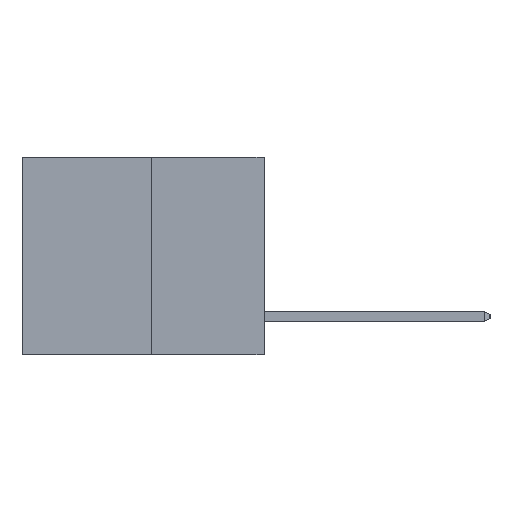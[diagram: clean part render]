
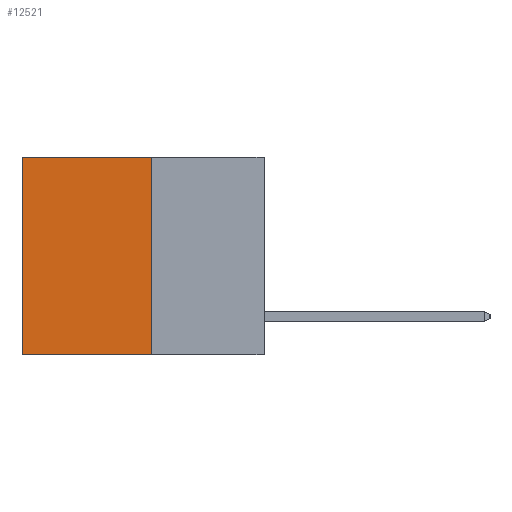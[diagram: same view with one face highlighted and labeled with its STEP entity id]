
A CAD part, left-side view. The second image highlights one B-rep face of the part: STEP entity #12521.
In plain terms, the highlighted planar face has unit normal (-1, 0, 0).
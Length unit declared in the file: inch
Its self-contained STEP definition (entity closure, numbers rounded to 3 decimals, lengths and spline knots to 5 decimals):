
#630 = DIRECTION ( 'NONE',  ( 1., 0., 0. ) ) ;
#1198 = CARTESIAN_POINT ( 'NONE',  ( 0.3165, 0.6, 0. ) ) ;
#1320 = EDGE_CURVE ( 'NONE', #2112, #13241, #15184, .T. ) ;
#1486 = CARTESIAN_POINT ( 'NONE',  ( 0.3165, 0.6, -0.49 ) ) ;
#2061 = DIRECTION ( 'NONE',  ( 0., 0., -1. ) ) ;
#2112 = VERTEX_POINT ( 'NONE', #1198 ) ;
#2833 = DIRECTION ( 'NONE',  ( 0., 1., 0. ) ) ;
#2996 = DIRECTION ( 'NONE',  ( 0., 0., -1. ) ) ;
#3142 = VERTEX_POINT ( 'NONE', #16560 ) ;
#4408 = EDGE_CURVE ( 'NONE', #3142, #2112, #5765, .T. ) ;
#5420 = CARTESIAN_POINT ( 'NONE',  ( 0.3165, 0.6, -0.49 ) ) ;
#5765 = LINE ( 'NONE', #13756, #8947 ) ;
#5780 = ORIENTED_EDGE ( 'NONE', *, *, #1320, .T. ) ;
#6660 = EDGE_CURVE ( 'NONE', #3142, #11105, #7778, .T. ) ;
#6782 = ORIENTED_EDGE ( 'NONE', *, *, #6660, .F. ) ;
#7140 = VECTOR ( 'NONE', #2061, 39.37008 ) ;
#7445 = AXIS2_PLACEMENT_3D ( 'NONE', #12868, #630, #7494 ) ;
#7494 = DIRECTION ( 'NONE',  ( 0., 0., -1. ) ) ;
#7778 = LINE ( 'NONE', #12800, #7140 ) ;
#8404 = VECTOR ( 'NONE', #2996, 39.37008 ) ;
#8504 = ORIENTED_EDGE ( 'NONE', *, *, #16594, .F. ) ;
#8947 = VECTOR ( 'NONE', #2833, 39.37008 ) ;
#9700 = VECTOR ( 'NONE', #10418, 39.37008 ) ;
#10418 = DIRECTION ( 'NONE',  ( 0., 1., 0. ) ) ;
#11105 = VERTEX_POINT ( 'NONE', #17344 ) ;
#11322 = PLANE ( 'NONE',  #7445 ) ;
#12407 = EDGE_LOOP ( 'NONE', ( #5780, #8504, #6782, #16929 ) ) ;
#12521 = ADVANCED_FACE ( 'NONE', ( #15545 ), #11322, .F. ) ;
#12800 = CARTESIAN_POINT ( 'NONE',  ( 0.3165, 0.28, -0.49 ) ) ;
#12868 = CARTESIAN_POINT ( 'NONE',  ( 0.3165, 0.28, -0.49 ) ) ;
#13241 = VERTEX_POINT ( 'NONE', #5420 ) ;
#13756 = CARTESIAN_POINT ( 'NONE',  ( 0.3165, 0.28, 0. ) ) ;
#15184 = LINE ( 'NONE', #1486, #8404 ) ;
#15545 = FACE_OUTER_BOUND ( 'NONE', #12407, .T. ) ;
#15619 = LINE ( 'NONE', #17259, #9700 ) ;
#16560 = CARTESIAN_POINT ( 'NONE',  ( 0.3165, 0.28, 0. ) ) ;
#16594 = EDGE_CURVE ( 'NONE', #11105, #13241, #15619, .T. ) ;
#16929 = ORIENTED_EDGE ( 'NONE', *, *, #4408, .T. ) ;
#17259 = CARTESIAN_POINT ( 'NONE',  ( 0.3165, 0.28, -0.49 ) ) ;
#17344 = CARTESIAN_POINT ( 'NONE',  ( 0.3165, 0.28, -0.49 ) ) ;
